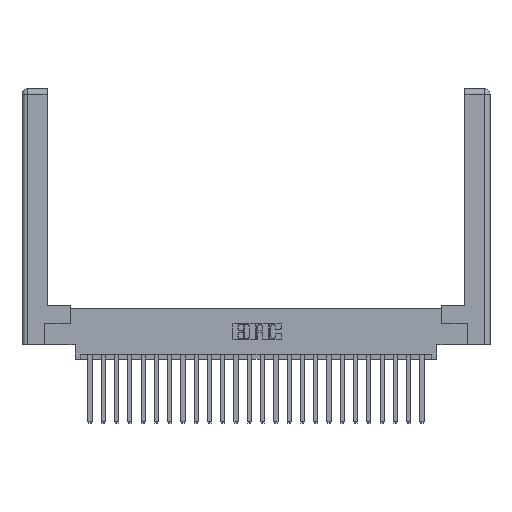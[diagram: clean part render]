
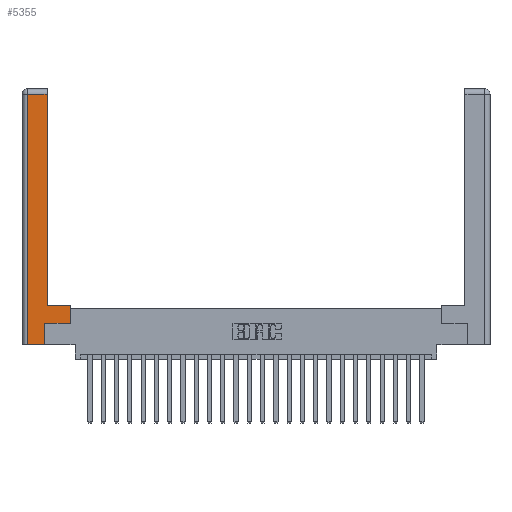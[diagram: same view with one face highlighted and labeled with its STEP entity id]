
A CAD part, top view. The second image highlights one B-rep face of the part: STEP entity #5355.
In plain terms, the highlighted planar face has unit normal (0, 0, 1).
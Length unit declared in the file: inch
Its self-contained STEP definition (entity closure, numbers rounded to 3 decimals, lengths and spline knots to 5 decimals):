
#200 = EDGE_CURVE ( 'NONE', #23157, #9795, #6227, .T. ) ;
#243 = CARTESIAN_POINT ( 'NONE',  ( 0.565, 0.245, 0. ) ) ;
#327 = ORIENTED_EDGE ( 'NONE', *, *, #5352, .T. ) ;
#895 = VECTOR ( 'NONE', #5925, 39.37008 ) ;
#967 = VECTOR ( 'NONE', #22603, 39.37008 ) ;
#1901 = LINE ( 'NONE', #3996, #23780 ) ;
#3875 = CARTESIAN_POINT ( 'NONE',  ( 0.565, 0.45, 0. ) ) ;
#3996 = CARTESIAN_POINT ( 'NONE',  ( 0.0615, 0., 0. ) ) ;
#5186 = CARTESIAN_POINT ( 'NONE',  ( 0.295, 2.94, 0. ) ) ;
#5255 = CARTESIAN_POINT ( 'NONE',  ( 0.0615, 2.94, 0. ) ) ;
#5317 = ORIENTED_EDGE ( 'NONE', *, *, #17149, .T. ) ;
#5352 = EDGE_CURVE ( 'NONE', #22293, #23157, #18125, .T. ) ;
#5355 = ADVANCED_FACE ( 'NONE', ( #18415 ), #20536, .F. ) ;
#5718 = LINE ( 'NONE', #6396, #24297 ) ;
#5925 = DIRECTION ( 'NONE',  ( 0., 1., 0. ) ) ;
#6227 = LINE ( 'NONE', #24787, #895 ) ;
#6396 = CARTESIAN_POINT ( 'NONE',  ( 0.0615, 2.94, 0. ) ) ;
#7139 = EDGE_CURVE ( 'NONE', #14880, #22293, #1901, .T. ) ;
#7423 = EDGE_CURVE ( 'NONE', #20273, #19514, #9960, .T. ) ;
#7476 = CARTESIAN_POINT ( 'NONE',  ( 0.265, 0.245, 0. ) ) ;
#7661 = DIRECTION ( 'NONE',  ( 0., 1., 0. ) ) ;
#8015 = ORIENTED_EDGE ( 'NONE', *, *, #7423, .T. ) ;
#8078 = AXIS2_PLACEMENT_3D ( 'NONE', #10780, #22466, #14574 ) ;
#8174 = VECTOR ( 'NONE', #13866, 39.37008 ) ;
#8318 = DIRECTION ( 'NONE',  ( -1., 0., 0. ) ) ;
#9641 = CARTESIAN_POINT ( 'NONE',  ( 0.295, 0.45, 0. ) ) ;
#9795 = VERTEX_POINT ( 'NONE', #7476 ) ;
#9960 = LINE ( 'NONE', #11786, #8174 ) ;
#10658 = CARTESIAN_POINT ( 'NONE',  ( 0.565, 0.45, 0. ) ) ;
#10780 = CARTESIAN_POINT ( 'NONE',  ( 0., 0., 0. ) ) ;
#10905 = EDGE_CURVE ( 'NONE', #19514, #14880, #5718, .T. ) ;
#11185 = VECTOR ( 'NONE', #20952, 39.37008 ) ;
#11238 = VERTEX_POINT ( 'NONE', #243 ) ;
#11495 = CARTESIAN_POINT ( 'NONE',  ( 0.265, 0., 0. ) ) ;
#11786 = CARTESIAN_POINT ( 'NONE',  ( 0.295, 3., 0. ) ) ;
#12342 = LINE ( 'NONE', #9641, #16592 ) ;
#12589 = CARTESIAN_POINT ( 'NONE',  ( 0.295, 0.45, 0. ) ) ;
#13555 = EDGE_LOOP ( 'NONE', ( #8015, #19226, #18857, #327, #22424, #17113, #5317, #23705 ) ) ;
#13589 = DIRECTION ( 'NONE',  ( -1., 0., 0. ) ) ;
#13866 = DIRECTION ( 'NONE',  ( 0., 1., 0. ) ) ;
#14574 = DIRECTION ( 'NONE',  ( -1., 0., 0. ) ) ;
#14880 = VERTEX_POINT ( 'NONE', #5255 ) ;
#16000 = CARTESIAN_POINT ( 'NONE',  ( 0.0615, 0., 0. ) ) ;
#16592 = VECTOR ( 'NONE', #13589, 39.37008 ) ;
#16890 = VERTEX_POINT ( 'NONE', #10658 ) ;
#17103 = LINE ( 'NONE', #3875, #19197 ) ;
#17113 = ORIENTED_EDGE ( 'NONE', *, *, #20301, .T. ) ;
#17130 = CARTESIAN_POINT ( 'NONE',  ( 0.265, 0., 0. ) ) ;
#17149 = EDGE_CURVE ( 'NONE', #11238, #16890, #17103, .T. ) ;
#17959 = DIRECTION ( 'NONE',  ( 0., -1., 0. ) ) ;
#18125 = LINE ( 'NONE', #17130, #11185 ) ;
#18415 = FACE_OUTER_BOUND ( 'NONE', #13555, .T. ) ;
#18763 = CARTESIAN_POINT ( 'NONE',  ( 0.565, 0.245, 0. ) ) ;
#18857 = ORIENTED_EDGE ( 'NONE', *, *, #7139, .T. ) ;
#19197 = VECTOR ( 'NONE', #7661, 39.37008 ) ;
#19226 = ORIENTED_EDGE ( 'NONE', *, *, #10905, .T. ) ;
#19514 = VERTEX_POINT ( 'NONE', #5186 ) ;
#20273 = VERTEX_POINT ( 'NONE', #12589 ) ;
#20301 = EDGE_CURVE ( 'NONE', #9795, #11238, #24683, .T. ) ;
#20536 = PLANE ( 'NONE',  #8078 ) ;
#20553 = EDGE_CURVE ( 'NONE', #16890, #20273, #12342, .T. ) ;
#20952 = DIRECTION ( 'NONE',  ( 1., 0., 0. ) ) ;
#22293 = VERTEX_POINT ( 'NONE', #16000 ) ;
#22424 = ORIENTED_EDGE ( 'NONE', *, *, #200, .T. ) ;
#22466 = DIRECTION ( 'NONE',  ( 0., 0., -1. ) ) ;
#22603 = DIRECTION ( 'NONE',  ( 1., 0., 0. ) ) ;
#23157 = VERTEX_POINT ( 'NONE', #11495 ) ;
#23705 = ORIENTED_EDGE ( 'NONE', *, *, #20553, .T. ) ;
#23780 = VECTOR ( 'NONE', #17959, 39.37008 ) ;
#24297 = VECTOR ( 'NONE', #8318, 39.37008 ) ;
#24683 = LINE ( 'NONE', #18763, #967 ) ;
#24787 = CARTESIAN_POINT ( 'NONE',  ( 0.265, 0.245, 0. ) ) ;
